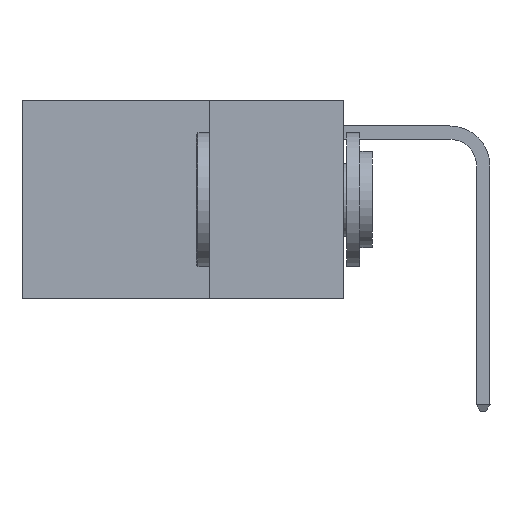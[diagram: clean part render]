
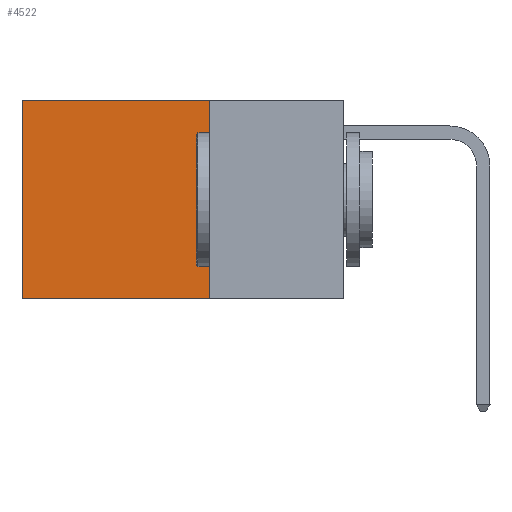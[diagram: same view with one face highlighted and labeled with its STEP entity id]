
A CAD part, left-side view. The second image highlights one B-rep face of the part: STEP entity #4522.
In plain terms, the highlighted planar face has unit normal (-1, 0, 0).
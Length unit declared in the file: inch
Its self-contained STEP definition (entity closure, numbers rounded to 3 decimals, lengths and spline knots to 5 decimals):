
#1422 = FACE_OUTER_BOUND ( 'NONE', #12633, .T. ) ;
#1469 = LINE ( 'NONE', #16210, #1500 ) ;
#1500 = VECTOR ( 'NONE', #16230, 39.37008 ) ;
#1835 = DIRECTION ( 'NONE',  ( 0., 0., -1. ) ) ;
#2008 = CARTESIAN_POINT ( 'NONE',  ( 0.2625, 0.25, 0. ) ) ;
#2721 = AXIS2_PLACEMENT_3D ( 'NONE', #8320, #8253, #8227 ) ;
#2723 = ORIENTED_EDGE ( 'NONE', *, *, #6620, .T. ) ;
#3495 = CARTESIAN_POINT ( 'NONE',  ( 0.2625, 0.6, -0.37 ) ) ;
#3604 = ORIENTED_EDGE ( 'NONE', *, *, #5170, .F. ) ;
#4522 = ADVANCED_FACE ( 'NONE', ( #1422 ), #8335, .F. ) ;
#4836 = LINE ( 'NONE', #5275, #11597 ) ;
#5002 = VERTEX_POINT ( 'NONE', #3495 ) ;
#5170 = EDGE_CURVE ( 'NONE', #15773, #5413, #16263, .T. ) ;
#5275 = CARTESIAN_POINT ( 'NONE',  ( 0.2625, 0.6, 0. ) ) ;
#5413 = VERTEX_POINT ( 'NONE', #12300 ) ;
#5662 = VERTEX_POINT ( 'NONE', #10639 ) ;
#6620 = EDGE_CURVE ( 'NONE', #15773, #5662, #8393, .T. ) ;
#8131 = VECTOR ( 'NONE', #14214, 39.37008 ) ;
#8227 = DIRECTION ( 'NONE',  ( 0., 0., -1. ) ) ;
#8253 = DIRECTION ( 'NONE',  ( 1., 0., 0. ) ) ;
#8320 = CARTESIAN_POINT ( 'NONE',  ( 0.2625, 0.25, 0. ) ) ;
#8335 = PLANE ( 'NONE',  #2721 ) ;
#8393 = LINE ( 'NONE', #14580, #8131 ) ;
#8786 = ORIENTED_EDGE ( 'NONE', *, *, #16329, .T. ) ;
#10129 = EDGE_CURVE ( 'NONE', #5413, #5002, #1469, .T. ) ;
#10639 = CARTESIAN_POINT ( 'NONE',  ( 0.2625, 0.6, 0. ) ) ;
#10645 = CARTESIAN_POINT ( 'NONE',  ( 0.2625, 0.25, 0. ) ) ;
#11597 = VECTOR ( 'NONE', #13313, 39.37008 ) ;
#12300 = CARTESIAN_POINT ( 'NONE',  ( 0.2625, 0.25, -0.37 ) ) ;
#12633 = EDGE_LOOP ( 'NONE', ( #8786, #15514, #3604, #2723 ) ) ;
#13313 = DIRECTION ( 'NONE',  ( 0., 0., -1. ) ) ;
#14214 = DIRECTION ( 'NONE',  ( 0., 1., 0. ) ) ;
#14580 = CARTESIAN_POINT ( 'NONE',  ( 0.2625, 0.25, 0. ) ) ;
#15514 = ORIENTED_EDGE ( 'NONE', *, *, #10129, .F. ) ;
#15773 = VERTEX_POINT ( 'NONE', #10645 ) ;
#16053 = VECTOR ( 'NONE', #1835, 39.37008 ) ;
#16210 = CARTESIAN_POINT ( 'NONE',  ( 0.2625, 0.25, -0.37 ) ) ;
#16230 = DIRECTION ( 'NONE',  ( 0., 1., 0. ) ) ;
#16263 = LINE ( 'NONE', #2008, #16053 ) ;
#16329 = EDGE_CURVE ( 'NONE', #5662, #5002, #4836, .T. ) ;
